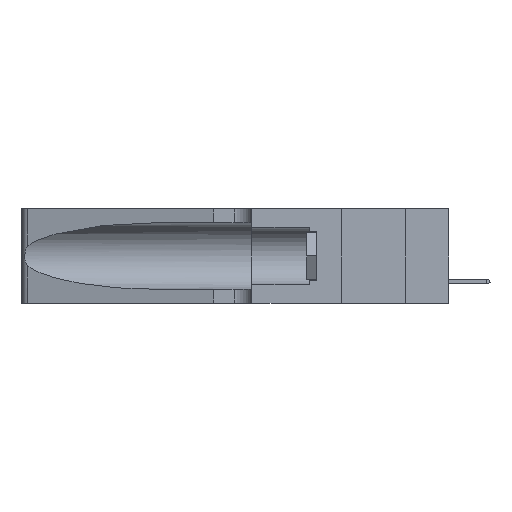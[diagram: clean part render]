
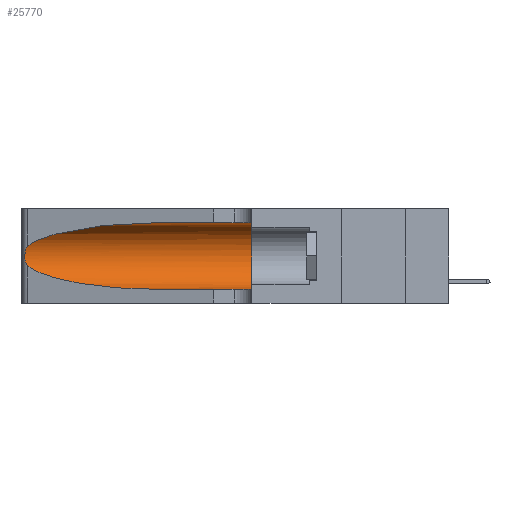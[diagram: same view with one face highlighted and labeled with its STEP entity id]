
A CAD part, left-side view. The second image highlights one B-rep face of the part: STEP entity #25770.
In plain terms, the highlighted cylindrical face has radius 3.308 mm (diameter 6.617 mm), a partial arc.
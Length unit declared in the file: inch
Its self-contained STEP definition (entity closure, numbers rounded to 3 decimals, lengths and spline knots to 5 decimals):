
#121 = EDGE_CURVE ( 'NONE', #32439, #13993, #36033, .T. ) ;
#2349 = VECTOR ( 'NONE', #21627, 39.37008 ) ;
#3457 = DIRECTION ( 'NONE',  ( 0., -1., 0. ) ) ;
#4465 = ORIENTED_EDGE ( 'NONE', *, *, #34312, .T. ) ;
#4470 = CARTESIAN_POINT ( 'NONE',  ( 0.26017, 1.23833, 0.17102 ) ) ;
#4600 = CARTESIAN_POINT ( 'NONE',  ( 0.25639, 1.23186, 0.15144 ) ) ;
#5686 = CARTESIAN_POINT ( 'NONE',  ( 0.18966, 0.96281, 0.05475 ) ) ;
#5796 = VERTEX_POINT ( 'NONE', #17096 ) ;
#7643 = CARTESIAN_POINT ( 'NONE',  ( 0.25487, 1.22718, 0.22369 ) ) ;
#7767 = CARTESIAN_POINT ( 'NONE',  ( 0.25789, 1.23486, 0.15765 ) ) ;
#9250 = VERTEX_POINT ( 'NONE', #33513 ) ;
#9345 = B_SPLINE_CURVE_WITH_KNOTS ( 'NONE', 3,
 ( #7643, #36882, #19194, #10544, #22146, #36513, #33796, #21905, #4470, #24837, #7767, #4600, #33676, #19427 ),
 .UNSPECIFIED., .F., .F.,
 ( 4, 2, 2, 2, 2, 2, 4 ),
 ( 0., 0.00027, 0.00053, 0.00107, 0.0016, 0.00187, 0.00214 ),
 .UNSPECIFIED. ) ;
#9634 = ORIENTED_EDGE ( 'NONE', *, *, #13007, .T. ) ;
#9872 = VERTEX_POINT ( 'NONE', #35380 ) ;
#10544 = CARTESIAN_POINT ( 'NONE',  ( 0.25787, 1.23484, 0.2124 ) ) ;
#11759 = CARTESIAN_POINT ( 'NONE',  ( 0.1305, 0.72297, 0.05475 ) ) ;
#13007 = EDGE_CURVE ( 'NONE', #5796, #9872, #18914, .T. ) ;
#13993 = VERTEX_POINT ( 'NONE', #23928 ) ;
#14871 = CARTESIAN_POINT ( 'NONE',  ( 0.1305, 1.61858, 0.185 ) ) ;
#15005 = DIRECTION ( 'NONE',  ( 0., 0., -1. ) ) ;
#16067 = FACE_OUTER_BOUND ( 'NONE', #34309, .T. ) ;
#16385 = CARTESIAN_POINT ( 'NONE',  ( 0.1305, 1.61858, 0.31525 ) ) ;
#16844 = LINE ( 'NONE', #16385, #27803 ) ;
#17096 = CARTESIAN_POINT ( 'NONE',  ( 0.1305, 0.72297, 0.31525 ) ) ;
#17631 = CARTESIAN_POINT ( 'NONE',  ( 0.1305, 0.72297, 0.05475 ) ) ;
#17778 = CARTESIAN_POINT ( 'NONE',  ( 0.18966, 0.96281, 0.31525 ) ) ;
#17954 = CIRCLE ( 'NONE', #32066, 0.13025 ) ;
#18042 = CARTESIAN_POINT ( 'NONE',  ( 0.1305, 0.72297, 0.31525 ) ) ;
#18353 = CYLINDRICAL_SURFACE ( 'NONE', #22007, 0.13025 ) ;
#18430 =( BOUNDED_CURVE ( )  B_SPLINE_CURVE ( 3, ( #19950, #22279, #5686, #11759 ),
 .UNSPECIFIED., .F., .F. ) 
 B_SPLINE_CURVE_WITH_KNOTS ( ( 4, 4 ),
 ( 3.44316, 4.71239 ),
 .UNSPECIFIED. ) 
 CURVE ( )  GEOMETRIC_REPRESENTATION_ITEM ( )  RATIONAL_B_SPLINE_CURVE ( ( 1., 0.87, 0.87, 1. ) ) 
 REPRESENTATION_ITEM ( '' )  );
#18684 = CARTESIAN_POINT ( 'NONE',  ( 0.1305, 1.61858, 0.05475 ) ) ;
#18914 =( BOUNDED_CURVE ( )  B_SPLINE_CURVE ( 3, ( #18042, #17778, #29758, #21227 ),
 .UNSPECIFIED., .F., .F. ) 
 B_SPLINE_CURVE_WITH_KNOTS ( ( 4, 4 ),
 ( 1.5708, 2.84003 ),
 .UNSPECIFIED. ) 
 CURVE ( )  GEOMETRIC_REPRESENTATION_ITEM ( )  RATIONAL_B_SPLINE_CURVE ( ( 1., 0.87, 0.87, 1. ) ) 
 REPRESENTATION_ITEM ( '' )  );
#18947 = EDGE_CURVE ( 'NONE', #5796, #9250, #16844, .T. ) ;
#19194 = CARTESIAN_POINT ( 'NONE',  ( 0.25639, 1.23184, 0.21858 ) ) ;
#19427 = CARTESIAN_POINT ( 'NONE',  ( 0.25487, 1.22718, 0.14631 ) ) ;
#19950 = CARTESIAN_POINT ( 'NONE',  ( 0.25487, 1.22718, 0.14631 ) ) ;
#21141 = VERTEX_POINT ( 'NONE', #36998 ) ;
#21227 = CARTESIAN_POINT ( 'NONE',  ( 0.25487, 1.22718, 0.22369 ) ) ;
#21627 = DIRECTION ( 'NONE',  ( 0., -1., 0. ) ) ;
#21905 = CARTESIAN_POINT ( 'NONE',  ( 0.26075, 1.23896, 0.178 ) ) ;
#22007 = AXIS2_PLACEMENT_3D ( 'NONE', #14871, #3457, #15005 ) ;
#22146 = CARTESIAN_POINT ( 'NONE',  ( 0.25854, 1.2359, 0.20912 ) ) ;
#22265 = DIRECTION ( 'NONE',  ( 0., -1., 0. ) ) ;
#22279 = CARTESIAN_POINT ( 'NONE',  ( 0.2373, 1.15595, 0.08982 ) ) ;
#23428 = DIRECTION ( 'NONE',  ( 0., 0., 1. ) ) ;
#23675 = CARTESIAN_POINT ( 'NONE',  ( 0.1305, 0.35, 0.185 ) ) ;
#23928 = CARTESIAN_POINT ( 'NONE',  ( 0.1305, 0.35, 0.05475 ) ) ;
#24257 = ORIENTED_EDGE ( 'NONE', *, *, #26139, .T. ) ;
#24335 = ORIENTED_EDGE ( 'NONE', *, *, #18947, .F. ) ;
#24837 = CARTESIAN_POINT ( 'NONE',  ( 0.25856, 1.23593, 0.16098 ) ) ;
#25770 = ADVANCED_FACE ( 'NONE', ( #16067 ), #18353, .F. ) ;
#26139 = EDGE_CURVE ( 'NONE', #9872, #21141, #9345, .T. ) ;
#26610 = DIRECTION ( 'NONE',  ( 0., 1., 0. ) ) ;
#27803 = VECTOR ( 'NONE', #22265, 39.37008 ) ;
#29758 = CARTESIAN_POINT ( 'NONE',  ( 0.2373, 1.15595, 0.28018 ) ) ;
#31571 = ORIENTED_EDGE ( 'NONE', *, *, #33624, .F. ) ;
#32066 = AXIS2_PLACEMENT_3D ( 'NONE', #23675, #26610, #23428 ) ;
#32439 = VERTEX_POINT ( 'NONE', #17631 ) ;
#32456 = ORIENTED_EDGE ( 'NONE', *, *, #121, .T. ) ;
#33513 = CARTESIAN_POINT ( 'NONE',  ( 0.1305, 0.35, 0.31525 ) ) ;
#33624 = EDGE_CURVE ( 'NONE', #9250, #13993, #17954, .T. ) ;
#33676 = CARTESIAN_POINT ( 'NONE',  ( 0.25555, 1.22993, 0.14849 ) ) ;
#33796 = CARTESIAN_POINT ( 'NONE',  ( 0.26075, 1.23896, 0.19203 ) ) ;
#34309 = EDGE_LOOP ( 'NONE', ( #9634, #24257, #4465, #32456, #31571, #24335 ) ) ;
#34312 = EDGE_CURVE ( 'NONE', #21141, #32439, #18430, .T. ) ;
#35380 = CARTESIAN_POINT ( 'NONE',  ( 0.25487, 1.22718, 0.22369 ) ) ;
#36033 = LINE ( 'NONE', #18684, #2349 ) ;
#36513 = CARTESIAN_POINT ( 'NONE',  ( 0.26018, 1.23835, 0.19895 ) ) ;
#36882 = CARTESIAN_POINT ( 'NONE',  ( 0.25555, 1.22994, 0.2215 ) ) ;
#36998 = CARTESIAN_POINT ( 'NONE',  ( 0.25487, 1.22718, 0.14631 ) ) ;
